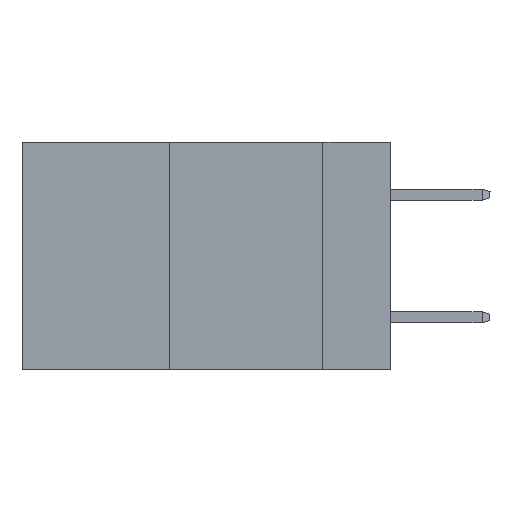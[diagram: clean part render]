
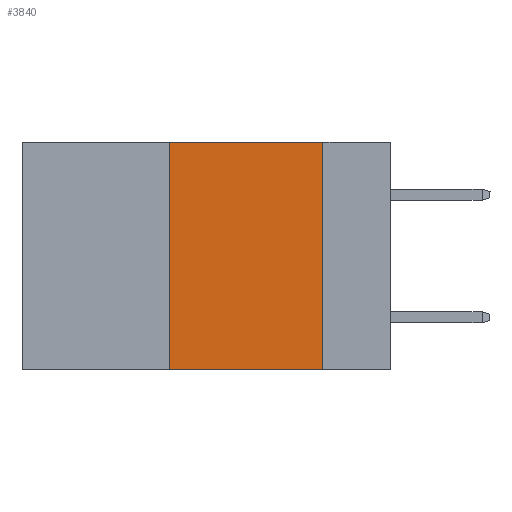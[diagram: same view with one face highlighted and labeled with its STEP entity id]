
A CAD part, left-side view. The second image highlights one B-rep face of the part: STEP entity #3840.
In plain terms, the highlighted planar face has unit normal (-1, 0, 0).
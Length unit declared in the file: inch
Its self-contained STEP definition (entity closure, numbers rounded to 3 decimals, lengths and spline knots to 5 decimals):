
#652 = VECTOR ( 'NONE', #11448, 39.37008 ) ;
#2671 = CARTESIAN_POINT ( 'NONE',  ( 0., 0.6, -0.37 ) ) ;
#3361 = FACE_OUTER_BOUND ( 'NONE', #11124, .T. ) ;
#3469 = ORIENTED_EDGE ( 'NONE', *, *, #9227, .F. ) ;
#3756 = DIRECTION ( 'NONE',  ( 1., 0., 0. ) ) ;
#3840 = ADVANCED_FACE ( 'NONE', ( #3361 ), #8818, .F. ) ;
#4061 = EDGE_CURVE ( 'NONE', #15843, #17707, #13215, .T. ) ;
#5122 = EDGE_CURVE ( 'NONE', #14191, #17707, #20407, .T. ) ;
#5555 = CARTESIAN_POINT ( 'NONE',  ( 0., 0.36, 0. ) ) ;
#6204 = CARTESIAN_POINT ( 'NONE',  ( 0., 0.36, 0. ) ) ;
#6331 = VERTEX_POINT ( 'NONE', #6204 ) ;
#8628 = ORIENTED_EDGE ( 'NONE', *, *, #17239, .F. ) ;
#8750 = LINE ( 'NONE', #5555, #11720 ) ;
#8818 = PLANE ( 'NONE',  #15857 ) ;
#8931 = VECTOR ( 'NONE', #21598, 39.37008 ) ;
#8979 = DIRECTION ( 'NONE',  ( 0., 0., 1. ) ) ;
#9143 = ORIENTED_EDGE ( 'NONE', *, *, #4061, .T. ) ;
#9227 = EDGE_CURVE ( 'NONE', #15843, #6331, #8750, .T. ) ;
#10551 = DIRECTION ( 'NONE',  ( 0., 0., -1. ) ) ;
#11124 = EDGE_LOOP ( 'NONE', ( #15007, #8628, #3469, #9143 ) ) ;
#11448 = DIRECTION ( 'NONE',  ( 0., -1., 0. ) ) ;
#11567 = CARTESIAN_POINT ( 'NONE',  ( 0., 0.11, -0.37 ) ) ;
#11620 = CARTESIAN_POINT ( 'NONE',  ( 0., 0.11, 0. ) ) ;
#11720 = VECTOR ( 'NONE', #8979, 39.37008 ) ;
#11856 = LINE ( 'NONE', #21371, #652 ) ;
#13215 = LINE ( 'NONE', #2671, #19079 ) ;
#14033 = CARTESIAN_POINT ( 'NONE',  ( 0., 0.6, 0. ) ) ;
#14191 = VERTEX_POINT ( 'NONE', #14573 ) ;
#14573 = CARTESIAN_POINT ( 'NONE',  ( 0., 0.11, 0. ) ) ;
#15007 = ORIENTED_EDGE ( 'NONE', *, *, #5122, .F. ) ;
#15843 = VERTEX_POINT ( 'NONE', #19576 ) ;
#15857 = AXIS2_PLACEMENT_3D ( 'NONE', #14033, #3756, #10551 ) ;
#17239 = EDGE_CURVE ( 'NONE', #6331, #14191, #11856, .T. ) ;
#17707 = VERTEX_POINT ( 'NONE', #11567 ) ;
#18157 = DIRECTION ( 'NONE',  ( 0., -1., 0. ) ) ;
#19079 = VECTOR ( 'NONE', #18157, 39.37008 ) ;
#19576 = CARTESIAN_POINT ( 'NONE',  ( 0., 0.36, -0.37 ) ) ;
#20407 = LINE ( 'NONE', #11620, #8931 ) ;
#21371 = CARTESIAN_POINT ( 'NONE',  ( 0., 0.6, 0. ) ) ;
#21598 = DIRECTION ( 'NONE',  ( 0., 0., -1. ) ) ;
